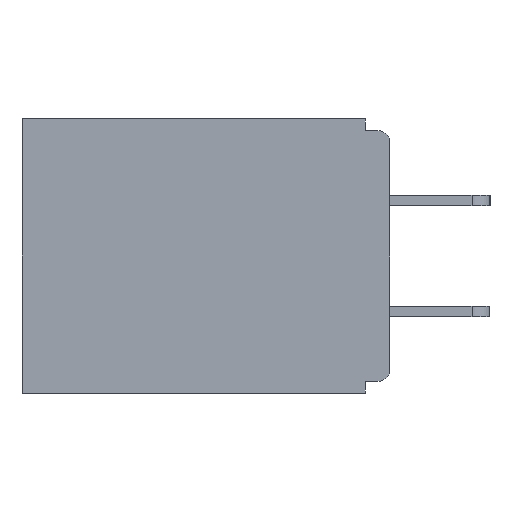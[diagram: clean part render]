
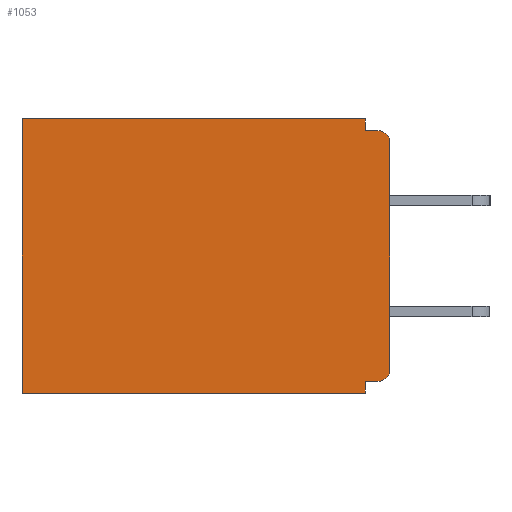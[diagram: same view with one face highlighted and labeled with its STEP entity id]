
A CAD part, left-side view. The second image highlights one B-rep face of the part: STEP entity #1053.
In plain terms, the highlighted planar face has unit normal (-1, 0, 0).
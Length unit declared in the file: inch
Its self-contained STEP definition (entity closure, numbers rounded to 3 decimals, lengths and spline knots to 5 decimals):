
#21 = VECTOR ( 'NONE', #9330, 39.37008 ) ;
#83 = DIRECTION ( 'NONE',  ( 0., 0., -1. ) ) ;
#219 = CARTESIAN_POINT ( 'NONE',  ( 0.298, 0., 0. ) ) ;
#244 = ORIENTED_EDGE ( 'NONE', *, *, #5762, .T. ) ;
#388 = VERTEX_POINT ( 'NONE', #11069 ) ;
#433 = ORIENTED_EDGE ( 'NONE', *, *, #660, .T. ) ;
#463 = DIRECTION ( 'NONE',  ( -1., 0., 0. ) ) ;
#660 = EDGE_CURVE ( 'NONE', #7050, #1740, #7810, .T. ) ;
#950 = VECTOR ( 'NONE', #10896, 39.37008 ) ;
#978 = PLANE ( 'NONE',  #6972 ) ;
#1010 = VERTEX_POINT ( 'NONE', #9886 ) ;
#1053 = ADVANCED_FACE ( 'NONE', ( #5053 ), #978, .F. ) ;
#1190 = EDGE_CURVE ( 'NONE', #5020, #7485, #7799, .T. ) ;
#1365 = CARTESIAN_POINT ( 'NONE',  ( 0.298, 0.031, -0.343 ) ) ;
#1740 = VERTEX_POINT ( 'NONE', #9574 ) ;
#1810 = CARTESIAN_POINT ( 'NONE',  ( 0.298, 0.031, 0. ) ) ;
#2164 = VECTOR ( 'NONE', #4202, 39.37008 ) ;
#2199 = CIRCLE ( 'NONE', #8730, 0.015 ) ;
#2207 = VECTOR ( 'NONE', #8332, 39.37008 ) ;
#2410 = ORIENTED_EDGE ( 'NONE', *, *, #6940, .F. ) ;
#2456 = LINE ( 'NONE', #10854, #2164 ) ;
#2468 = ORIENTED_EDGE ( 'NONE', *, *, #11035, .F. ) ;
#2502 = VECTOR ( 'NONE', #8699, 39.37008 ) ;
#2661 = DIRECTION ( 'NONE',  ( 0., 0., -1. ) ) ;
#2719 = DIRECTION ( 'NONE',  ( 1., 0., 0. ) ) ;
#2842 = CARTESIAN_POINT ( 'NONE',  ( 0.298, 0., 0. ) ) ;
#2908 = VERTEX_POINT ( 'NONE', #4714 ) ;
#3125 = CARTESIAN_POINT ( 'NONE',  ( 0.298, 0.015, -0.313 ) ) ;
#3357 = VECTOR ( 'NONE', #10737, 39.37008 ) ;
#3508 = LINE ( 'NONE', #3615, #3357 ) ;
#3615 = CARTESIAN_POINT ( 'NONE',  ( 0.298, 0., -0.015 ) ) ;
#4005 = CARTESIAN_POINT ( 'NONE',  ( 0.298, 0.015, -0.03 ) ) ;
#4087 = EDGE_CURVE ( 'NONE', #6394, #9890, #7276, .T. ) ;
#4202 = DIRECTION ( 'NONE',  ( 0., 0., -1. ) ) ;
#4233 = CARTESIAN_POINT ( 'NONE',  ( 0.298, 0., -0.03 ) ) ;
#4714 = CARTESIAN_POINT ( 'NONE',  ( 0.298, 0.015, -0.328 ) ) ;
#4738 = ORIENTED_EDGE ( 'NONE', *, *, #9354, .F. ) ;
#4831 = CARTESIAN_POINT ( 'NONE',  ( 0.298, 0., -0.343 ) ) ;
#4863 = ORIENTED_EDGE ( 'NONE', *, *, #5775, .T. ) ;
#5014 = VERTEX_POINT ( 'NONE', #1810 ) ;
#5020 = VERTEX_POINT ( 'NONE', #7068 ) ;
#5053 = FACE_OUTER_BOUND ( 'NONE', #6025, .T. ) ;
#5320 = LINE ( 'NONE', #219, #5875 ) ;
#5431 = CARTESIAN_POINT ( 'NONE',  ( 0.298, 0.46, 0. ) ) ;
#5739 = LINE ( 'NONE', #11080, #21 ) ;
#5762 = EDGE_CURVE ( 'NONE', #2908, #388, #2199, .T. ) ;
#5767 = DIRECTION ( 'NONE',  ( 0., 0., -1. ) ) ;
#5775 = EDGE_CURVE ( 'NONE', #5014, #6394, #5739, .T. ) ;
#5875 = VECTOR ( 'NONE', #2661, 39.37008 ) ;
#6025 = EDGE_LOOP ( 'NONE', ( #433, #4738, #2410, #4863, #7711, #2468, #10218, #7546, #244, #6907 ) ) ;
#6394 = VERTEX_POINT ( 'NONE', #9395 ) ;
#6608 = CARTESIAN_POINT ( 'NONE',  ( 0.298, 0.031, -0.343 ) ) ;
#6651 = CARTESIAN_POINT ( 'NONE',  ( 0.298, 0.46, -0.343 ) ) ;
#6696 = DIRECTION ( 'NONE',  ( -1., 0., 0. ) ) ;
#6907 = ORIENTED_EDGE ( 'NONE', *, *, #9511, .F. ) ;
#6940 = EDGE_CURVE ( 'NONE', #5014, #1010, #2456, .T. ) ;
#6972 = AXIS2_PLACEMENT_3D ( 'NONE', #2842, #2719, #7298 ) ;
#7050 = VERTEX_POINT ( 'NONE', #4233 ) ;
#7068 = CARTESIAN_POINT ( 'NONE',  ( 0.298, 0.031, -0.328 ) ) ;
#7276 = LINE ( 'NONE', #5431, #9440 ) ;
#7298 = DIRECTION ( 'NONE',  ( 0., 0., -1. ) ) ;
#7485 = VERTEX_POINT ( 'NONE', #1365 ) ;
#7546 = ORIENTED_EDGE ( 'NONE', *, *, #9143, .F. ) ;
#7711 = ORIENTED_EDGE ( 'NONE', *, *, #4087, .T. ) ;
#7799 = LINE ( 'NONE', #6608, #2207 ) ;
#7810 = CIRCLE ( 'NONE', #9011, 0.015 ) ;
#8332 = DIRECTION ( 'NONE',  ( 0., 0., -1. ) ) ;
#8699 = DIRECTION ( 'NONE',  ( 0., 1., 0. ) ) ;
#8730 = AXIS2_PLACEMENT_3D ( 'NONE', #3125, #6696, #5767 ) ;
#9011 = AXIS2_PLACEMENT_3D ( 'NONE', #4005, #463, #9237 ) ;
#9143 = EDGE_CURVE ( 'NONE', #2908, #5020, #10688, .T. ) ;
#9237 = DIRECTION ( 'NONE',  ( 0., 0., -1. ) ) ;
#9330 = DIRECTION ( 'NONE',  ( 0., 1., 0. ) ) ;
#9354 = EDGE_CURVE ( 'NONE', #1010, #1740, #3508, .T. ) ;
#9395 = CARTESIAN_POINT ( 'NONE',  ( 0.298, 0.46, 0. ) ) ;
#9440 = VECTOR ( 'NONE', #83, 39.37008 ) ;
#9511 = EDGE_CURVE ( 'NONE', #7050, #388, #5320, .T. ) ;
#9574 = CARTESIAN_POINT ( 'NONE',  ( 0.298, 0.015, -0.015 ) ) ;
#9745 = CARTESIAN_POINT ( 'NONE',  ( 0.298, 0., -0.328 ) ) ;
#9886 = CARTESIAN_POINT ( 'NONE',  ( 0.298, 0.031, -0.015 ) ) ;
#9890 = VERTEX_POINT ( 'NONE', #6651 ) ;
#10218 = ORIENTED_EDGE ( 'NONE', *, *, #1190, .F. ) ;
#10688 = LINE ( 'NONE', #9745, #2502 ) ;
#10737 = DIRECTION ( 'NONE',  ( 0., -1., 0. ) ) ;
#10854 = CARTESIAN_POINT ( 'NONE',  ( 0.298, 0.031, -0.343 ) ) ;
#10896 = DIRECTION ( 'NONE',  ( 0., 1., 0. ) ) ;
#11035 = EDGE_CURVE ( 'NONE', #7485, #9890, #11049, .T. ) ;
#11049 = LINE ( 'NONE', #4831, #950 ) ;
#11069 = CARTESIAN_POINT ( 'NONE',  ( 0.298, 0., -0.313 ) ) ;
#11080 = CARTESIAN_POINT ( 'NONE',  ( 0.298, 0., 0. ) ) ;
